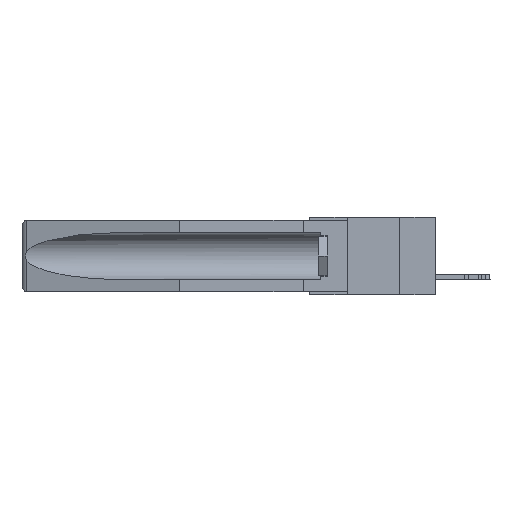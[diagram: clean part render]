
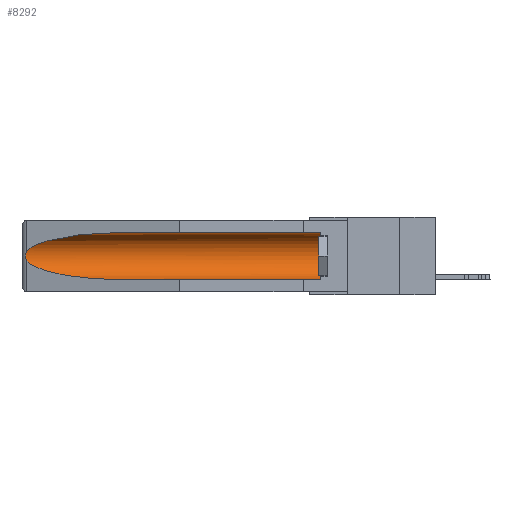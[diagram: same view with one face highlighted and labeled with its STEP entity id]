
A CAD part, left-side view. The second image highlights one B-rep face of the part: STEP entity #8292.
In plain terms, the highlighted cylindrical face has radius 2.857 mm (diameter 5.715 mm), a partial arc.
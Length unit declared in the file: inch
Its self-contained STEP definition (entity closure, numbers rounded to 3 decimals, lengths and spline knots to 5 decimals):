
#256 = DIRECTION ( 'NONE',  ( 0., 0., 1. ) ) ;
#317 = EDGE_CURVE ( 'NONE', #22485, #10136, #14986, .T. ) ;
#669 = CARTESIAN_POINT ( 'NONE',  ( 0.155, -0.30754, -0.284 ) ) ;
#708 =( BOUNDED_CURVE ( )  B_SPLINE_CURVE ( 3, ( #10257, #29095, #29205, #17041 ),
 .UNSPECIFIED., .F., .F. ) 
 B_SPLINE_CURVE_WITH_KNOTS ( ( 4, 4 ),
 ( 0.1948, 1.5708 ),
 .UNSPECIFIED. ) 
 CURVE ( )  GEOMETRIC_REPRESENTATION_ITEM ( )  RATIONAL_B_SPLINE_CURVE ( ( 1., 0.848, 0.848, 1. ) ) 
 REPRESENTATION_ITEM ( '' )  );
#1319 = VERTEX_POINT ( 'NONE', #16226 ) ;
#1834 = CARTESIAN_POINT ( 'NONE',  ( 0.26597, 1.5296, -0.19026 ) ) ;
#2218 = ORIENTED_EDGE ( 'NONE', *, *, #29567, .F. ) ;
#2396 = ORIENTED_EDGE ( 'NONE', *, *, #317, .T. ) ;
#2492 = ORIENTED_EDGE ( 'NONE', *, *, #4377, .T. ) ;
#3153 = EDGE_CURVE ( 'NONE', #1319, #22708, #708, .T. ) ;
#3299 = DIRECTION ( 'NONE',  ( 0., 0., 1. ) ) ;
#4377 = EDGE_CURVE ( 'NONE', #13484, #4664, #26154, .T. ) ;
#4664 = VERTEX_POINT ( 'NONE', #24565 ) ;
#5974 = CARTESIAN_POINT ( 'NONE',  ( 0.2673, 1.5327, -0.16383 ) ) ;
#6572 = CARTESIAN_POINT ( 'NONE',  ( 0.2673, 1.53269, -0.17917 ) ) ;
#7073 = CARTESIAN_POINT ( 'NONE',  ( 0.26537, 1.52718, -0.14972 ) ) ;
#8089 = B_SPLINE_CURVE_WITH_KNOTS ( 'NONE', 3,
 ( #27185, #15624, #29371, #5974, #13540, #18211, #6572, #11245, #1834, #11351 ),
 .UNSPECIFIED., .F., .F.,
 ( 4, 2, 2, 2, 4 ),
 ( 0., 0.00029, 0.00058, 0.00087, 0.00117 ),
 .UNSPECIFIED. ) ;
#8292 = ADVANCED_FACE ( 'NONE', ( #26670 ), #18909, .F. ) ;
#8363 = EDGE_LOOP ( 'NONE', ( #2396, #11848, #10574, #2218, #2492, #19158 ) ) ;
#9346 = DIRECTION ( 'NONE',  ( 0., -1., 0. ) ) ;
#9347 = CARTESIAN_POINT ( 'NONE',  ( 0.155, 1.07973, -0.059 ) ) ;
#10136 = VERTEX_POINT ( 'NONE', #27216 ) ;
#10257 = CARTESIAN_POINT ( 'NONE',  ( 0.26537, 1.52718, -0.19328 ) ) ;
#10574 = ORIENTED_EDGE ( 'NONE', *, *, #3153, .T. ) ;
#11245 = CARTESIAN_POINT ( 'NONE',  ( 0.26655, 1.53094, -0.18657 ) ) ;
#11289 = CARTESIAN_POINT ( 'NONE',  ( 0.155, 1.07973, -0.284 ) ) ;
#11351 = CARTESIAN_POINT ( 'NONE',  ( 0.26537, 1.52718, -0.19328 ) ) ;
#11383 = CARTESIAN_POINT ( 'NONE',  ( 0.155, 0.126, -0.284 ) ) ;
#11762 = CARTESIAN_POINT ( 'NONE',  ( 0.21114, 1.30732, -0.059 ) ) ;
#11848 = ORIENTED_EDGE ( 'NONE', *, *, #14174, .T. ) ;
#11910 = AXIS2_PLACEMENT_3D ( 'NONE', #19103, #9346, #256 ) ;
#12991 = VECTOR ( 'NONE', #14999, 39.37008 ) ;
#13162 = CARTESIAN_POINT ( 'NONE',  ( 0.155, 1.07973, -0.059 ) ) ;
#13358 = VECTOR ( 'NONE', #27585, 39.37008 ) ;
#13484 = VERTEX_POINT ( 'NONE', #11383 ) ;
#13540 = CARTESIAN_POINT ( 'NONE',  ( 0.2675, 1.53308, -0.16763 ) ) ;
#13638 = CARTESIAN_POINT ( 'NONE',  ( 0.155, -0.30754, -0.059 ) ) ;
#14174 = EDGE_CURVE ( 'NONE', #10136, #1319, #8089, .T. ) ;
#14187 = EDGE_CURVE ( 'NONE', #4664, #22485, #25136, .T. ) ;
#14986 =( BOUNDED_CURVE ( )  B_SPLINE_CURVE ( 3, ( #9347, #11762, #21288, #7073 ),
 .UNSPECIFIED., .F., .F. ) 
 B_SPLINE_CURVE_WITH_KNOTS ( ( 4, 4 ),
 ( 4.71239, 6.08839 ),
 .UNSPECIFIED. ) 
 CURVE ( )  GEOMETRIC_REPRESENTATION_ITEM ( )  RATIONAL_B_SPLINE_CURVE ( ( 1., 0.848, 0.848, 1. ) ) 
 REPRESENTATION_ITEM ( '' )  );
#14999 = DIRECTION ( 'NONE',  ( 0., 1., 0. ) ) ;
#15116 = DIRECTION ( 'NONE',  ( 0., 1., 0. ) ) ;
#15624 = CARTESIAN_POINT ( 'NONE',  ( 0.26597, 1.52961, -0.15275 ) ) ;
#16226 = CARTESIAN_POINT ( 'NONE',  ( 0.26537, 1.52718, -0.19328 ) ) ;
#16569 = AXIS2_PLACEMENT_3D ( 'NONE', #29253, #15116, #3299 ) ;
#17041 = CARTESIAN_POINT ( 'NONE',  ( 0.155, 1.07973, -0.284 ) ) ;
#18211 = CARTESIAN_POINT ( 'NONE',  ( 0.2675, 1.53308, -0.17534 ) ) ;
#18909 = CYLINDRICAL_SURFACE ( 'NONE', #16569, 0.1125 ) ;
#19103 = CARTESIAN_POINT ( 'NONE',  ( 0.155, 0.126, -0.1715 ) ) ;
#19158 = ORIENTED_EDGE ( 'NONE', *, *, #14187, .T. ) ;
#21288 = CARTESIAN_POINT ( 'NONE',  ( 0.25451, 1.48313, -0.09465 ) ) ;
#22485 = VERTEX_POINT ( 'NONE', #13162 ) ;
#22708 = VERTEX_POINT ( 'NONE', #11289 ) ;
#24565 = CARTESIAN_POINT ( 'NONE',  ( 0.155, 0.126, -0.059 ) ) ;
#25136 = LINE ( 'NONE', #13638, #13358 ) ;
#26154 = CIRCLE ( 'NONE', #11910, 0.1125 ) ;
#26670 = FACE_OUTER_BOUND ( 'NONE', #8363, .T. ) ;
#27185 = CARTESIAN_POINT ( 'NONE',  ( 0.26537, 1.52718, -0.14972 ) ) ;
#27216 = CARTESIAN_POINT ( 'NONE',  ( 0.26537, 1.52718, -0.14972 ) ) ;
#27585 = DIRECTION ( 'NONE',  ( 0., 1., 0. ) ) ;
#29095 = CARTESIAN_POINT ( 'NONE',  ( 0.25451, 1.48313, -0.24835 ) ) ;
#29205 = CARTESIAN_POINT ( 'NONE',  ( 0.21114, 1.30732, -0.284 ) ) ;
#29253 = CARTESIAN_POINT ( 'NONE',  ( 0.155, -0.30754, -0.1715 ) ) ;
#29371 = CARTESIAN_POINT ( 'NONE',  ( 0.26654, 1.53092, -0.15636 ) ) ;
#29567 = EDGE_CURVE ( 'NONE', #13484, #22708, #30393, .T. ) ;
#30393 = LINE ( 'NONE', #669, #12991 ) ;
